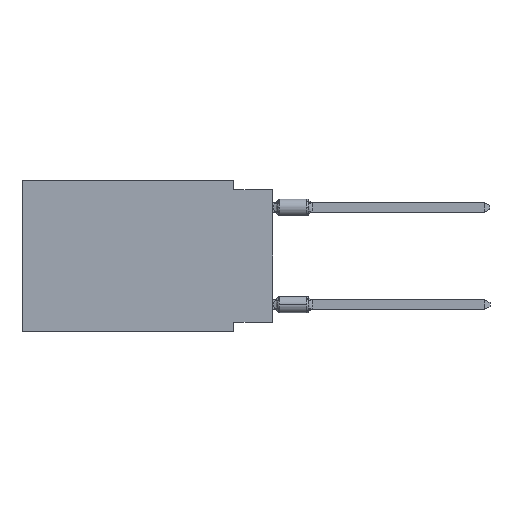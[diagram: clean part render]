
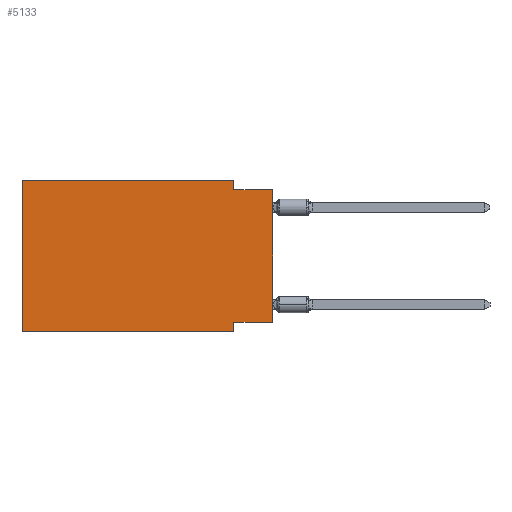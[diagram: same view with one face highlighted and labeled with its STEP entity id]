
A CAD part, left-side view. The second image highlights one B-rep face of the part: STEP entity #5133.
In plain terms, the highlighted planar face has unit normal (-1, 0, 0).
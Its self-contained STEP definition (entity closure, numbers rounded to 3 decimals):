
#73 = VECTOR ( 'NONE', #9294, 1000. ) ;
#137 = DIRECTION ( 'NONE',  ( 1., 0., 0. ) ) ;
#271 = CARTESIAN_POINT ( 'NONE',  ( 0., 0., -9.271 ) ) ;
#275 = ORIENTED_EDGE ( 'NONE', *, *, #14128, .T. ) ;
#468 = LINE ( 'NONE', #13609, #73 ) ;
#812 = CARTESIAN_POINT ( 'NONE',  ( 0., 0., -0.635 ) ) ;
#1279 = CARTESIAN_POINT ( 'NONE',  ( 0., 2.54, -0.635 ) ) ;
#1923 = LINE ( 'NONE', #13217, #7936 ) ;
#3005 = ORIENTED_EDGE ( 'NONE', *, *, #17664, .T. ) ;
#3303 = EDGE_CURVE ( 'NONE', #4708, #7486, #468, .T. ) ;
#3957 = CARTESIAN_POINT ( 'NONE',  ( 0., 2.54, 0. ) ) ;
#4275 = CARTESIAN_POINT ( 'NONE',  ( 0., 16.383, 0. ) ) ;
#4374 = LINE ( 'NONE', #14804, #5500 ) ;
#4708 = VERTEX_POINT ( 'NONE', #1279 ) ;
#4736 = VERTEX_POINT ( 'NONE', #11643 ) ;
#4777 = LINE ( 'NONE', #271, #18152 ) ;
#4999 = VECTOR ( 'NONE', #11610, 1000. ) ;
#5109 = CARTESIAN_POINT ( 'NONE',  ( 0., 2.54, 0. ) ) ;
#5133 = ADVANCED_FACE ( 'NONE', ( #8426 ), #10107, .F. ) ;
#5208 = EDGE_CURVE ( 'NONE', #14223, #5278, #1923, .T. ) ;
#5278 = VERTEX_POINT ( 'NONE', #5109 ) ;
#5290 = DIRECTION ( 'NONE',  ( 0., 0., -1. ) ) ;
#5500 = VECTOR ( 'NONE', #10104, 1000. ) ;
#6047 = LINE ( 'NONE', #12918, #4999 ) ;
#6059 = DIRECTION ( 'NONE',  ( 0., -1., 0. ) ) ;
#6184 = VECTOR ( 'NONE', #6847, 1000. ) ;
#6319 = DIRECTION ( 'NONE',  ( 0., 0., 1. ) ) ;
#6708 = VERTEX_POINT ( 'NONE', #17493 ) ;
#6847 = DIRECTION ( 'NONE',  ( 0., 0., 1. ) ) ;
#7270 = EDGE_CURVE ( 'NONE', #15650, #4736, #4777, .T. ) ;
#7486 = VERTEX_POINT ( 'NONE', #812 ) ;
#7729 = LINE ( 'NONE', #13470, #17547 ) ;
#7936 = VECTOR ( 'NONE', #6059, 1000. ) ;
#8426 = FACE_OUTER_BOUND ( 'NONE', #15913, .T. ) ;
#8735 = ORIENTED_EDGE ( 'NONE', *, *, #7270, .F. ) ;
#9205 = DIRECTION ( 'NONE',  ( 0., 1., 0. ) ) ;
#9294 = DIRECTION ( 'NONE',  ( 0., -1., 0. ) ) ;
#10104 = DIRECTION ( 'NONE',  ( 0., -1., 0. ) ) ;
#10107 = PLANE ( 'NONE',  #15770 ) ;
#10651 = EDGE_CURVE ( 'NONE', #4736, #6708, #6047, .T. ) ;
#10857 = EDGE_CURVE ( 'NONE', #5278, #4708, #12524, .T. ) ;
#11012 = VECTOR ( 'NONE', #5290, 1000. ) ;
#11610 = DIRECTION ( 'NONE',  ( 0., 0., -1. ) ) ;
#11643 = CARTESIAN_POINT ( 'NONE',  ( 0., 2.54, -9.271 ) ) ;
#11792 = ORIENTED_EDGE ( 'NONE', *, *, #14730, .F. ) ;
#12084 = ORIENTED_EDGE ( 'NONE', *, *, #10651, .F. ) ;
#12524 = LINE ( 'NONE', #3957, #11012 ) ;
#12604 = ORIENTED_EDGE ( 'NONE', *, *, #5208, .F. ) ;
#12814 = CARTESIAN_POINT ( 'NONE',  ( 0., 0., -9.271 ) ) ;
#12918 = CARTESIAN_POINT ( 'NONE',  ( 0., 2.54, -9.906 ) ) ;
#13217 = CARTESIAN_POINT ( 'NONE',  ( 0., 16.383, 0. ) ) ;
#13411 = VERTEX_POINT ( 'NONE', #15025 ) ;
#13470 = CARTESIAN_POINT ( 'NONE',  ( 0., 16.383, 0. ) ) ;
#13609 = CARTESIAN_POINT ( 'NONE',  ( 0., 0., -0.635 ) ) ;
#14128 = EDGE_CURVE ( 'NONE', #13411, #6708, #4374, .T. ) ;
#14223 = VERTEX_POINT ( 'NONE', #14628 ) ;
#14353 = DIRECTION ( 'NONE',  ( 0., 0., -1. ) ) ;
#14628 = CARTESIAN_POINT ( 'NONE',  ( 0., 16.383, 0. ) ) ;
#14730 = EDGE_CURVE ( 'NONE', #13411, #14223, #7729, .T. ) ;
#14804 = CARTESIAN_POINT ( 'NONE',  ( 0., 16.383, -9.906 ) ) ;
#14879 = ORIENTED_EDGE ( 'NONE', *, *, #3303, .F. ) ;
#15025 = CARTESIAN_POINT ( 'NONE',  ( 0., 16.383, -9.906 ) ) ;
#15650 = VERTEX_POINT ( 'NONE', #12814 ) ;
#15770 = AXIS2_PLACEMENT_3D ( 'NONE', #4275, #137, #14353 ) ;
#15913 = EDGE_LOOP ( 'NONE', ( #3005, #14879, #18166, #12604, #11792, #275, #12084, #8735 ) ) ;
#17088 = LINE ( 'NONE', #18380, #6184 ) ;
#17493 = CARTESIAN_POINT ( 'NONE',  ( 0., 2.54, -9.906 ) ) ;
#17547 = VECTOR ( 'NONE', #6319, 1000. ) ;
#17664 = EDGE_CURVE ( 'NONE', #15650, #7486, #17088, .T. ) ;
#18152 = VECTOR ( 'NONE', #9205, 1000. ) ;
#18166 = ORIENTED_EDGE ( 'NONE', *, *, #10857, .F. ) ;
#18380 = CARTESIAN_POINT ( 'NONE',  ( 0., 0., 0. ) ) ;
